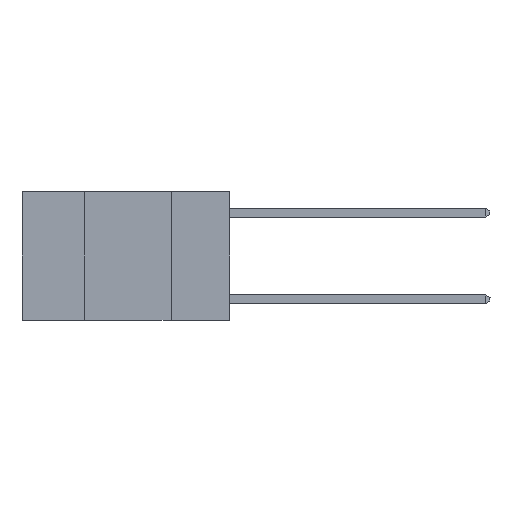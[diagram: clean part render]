
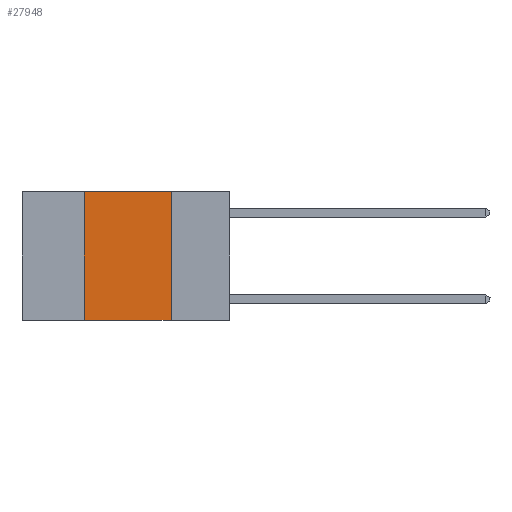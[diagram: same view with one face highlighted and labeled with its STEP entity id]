
A CAD part, left-side view. The second image highlights one B-rep face of the part: STEP entity #27948.
In plain terms, the highlighted planar face has unit normal (-1, 0, 0).
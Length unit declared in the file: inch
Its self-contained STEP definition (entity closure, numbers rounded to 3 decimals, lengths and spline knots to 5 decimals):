
#263 = VERTEX_POINT ( 'NONE', #4919 ) ;
#794 = LINE ( 'NONE', #28828, #5810 ) ;
#1094 = CARTESIAN_POINT ( 'NONE',  ( 0., 0.17, 0. ) ) ;
#2095 = CARTESIAN_POINT ( 'NONE',  ( 0., 0.6, -0.37 ) ) ;
#3523 = ORIENTED_EDGE ( 'NONE', *, *, #21087, .F. ) ;
#3570 = DIRECTION ( 'NONE',  ( 0., 0., -1. ) ) ;
#3709 = FACE_OUTER_BOUND ( 'NONE', #17691, .T. ) ;
#4905 = CARTESIAN_POINT ( 'NONE',  ( 0., 0.42, 0. ) ) ;
#4919 = CARTESIAN_POINT ( 'NONE',  ( 0., 0.17, -0.37 ) ) ;
#5810 = VECTOR ( 'NONE', #16570, 39.37008 ) ;
#7067 = AXIS2_PLACEMENT_3D ( 'NONE', #13591, #30787, #16052 ) ;
#7398 = DIRECTION ( 'NONE',  ( 0., 0., 1. ) ) ;
#7776 = CARTESIAN_POINT ( 'NONE',  ( 0., 0.17, 0. ) ) ;
#10907 = ORIENTED_EDGE ( 'NONE', *, *, #12412, .F. ) ;
#11118 = ORIENTED_EDGE ( 'NONE', *, *, #14963, .T. ) ;
#12104 = LINE ( 'NONE', #1094, #24427 ) ;
#12412 = EDGE_CURVE ( 'NONE', #24784, #30805, #794, .T. ) ;
#12609 = VECTOR ( 'NONE', #19377, 39.37008 ) ;
#13591 = CARTESIAN_POINT ( 'NONE',  ( 0., 0.6, 0. ) ) ;
#14490 = EDGE_CURVE ( 'NONE', #30732, #24784, #26504, .T. ) ;
#14963 = EDGE_CURVE ( 'NONE', #30732, #263, #18397, .T. ) ;
#16052 = DIRECTION ( 'NONE',  ( 0., 0., -1. ) ) ;
#16570 = DIRECTION ( 'NONE',  ( 0., -1., 0. ) ) ;
#17691 = EDGE_LOOP ( 'NONE', ( #3523, #10907, #26119, #11118 ) ) ;
#18397 = LINE ( 'NONE', #2095, #12609 ) ;
#19377 = DIRECTION ( 'NONE',  ( 0., -1., 0. ) ) ;
#20240 = CARTESIAN_POINT ( 'NONE',  ( 0., 0.42, 0. ) ) ;
#21087 = EDGE_CURVE ( 'NONE', #30805, #263, #12104, .T. ) ;
#24427 = VECTOR ( 'NONE', #3570, 39.37008 ) ;
#24784 = VERTEX_POINT ( 'NONE', #20240 ) ;
#24959 = VECTOR ( 'NONE', #7398, 39.37008 ) ;
#26119 = ORIENTED_EDGE ( 'NONE', *, *, #14490, .F. ) ;
#26504 = LINE ( 'NONE', #4905, #24959 ) ;
#27295 = CARTESIAN_POINT ( 'NONE',  ( 0., 0.42, -0.37 ) ) ;
#27948 = ADVANCED_FACE ( 'NONE', ( #3709 ), #28336, .F. ) ;
#28336 = PLANE ( 'NONE',  #7067 ) ;
#28828 = CARTESIAN_POINT ( 'NONE',  ( 0., 0.6, 0. ) ) ;
#30732 = VERTEX_POINT ( 'NONE', #27295 ) ;
#30787 = DIRECTION ( 'NONE',  ( 1., 0., 0. ) ) ;
#30805 = VERTEX_POINT ( 'NONE', #7776 ) ;
